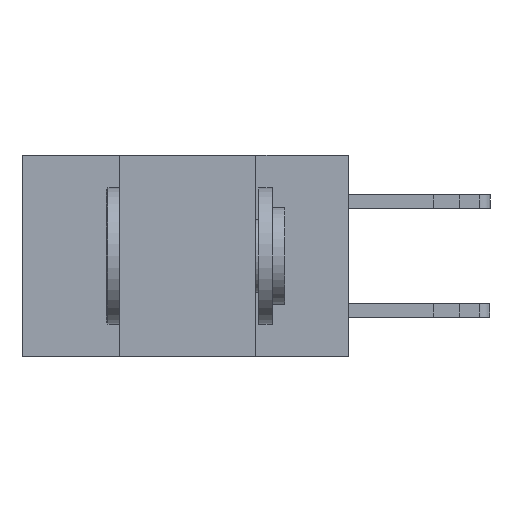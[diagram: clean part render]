
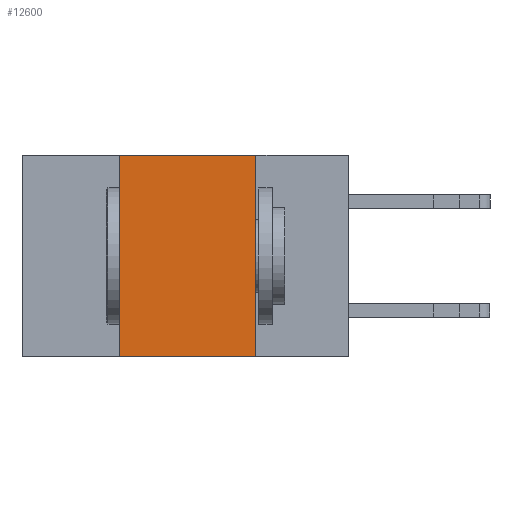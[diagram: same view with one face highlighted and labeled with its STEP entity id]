
A CAD part, left-side view. The second image highlights one B-rep face of the part: STEP entity #12600.
In plain terms, the highlighted planar face has unit normal (-1, 0, 0).
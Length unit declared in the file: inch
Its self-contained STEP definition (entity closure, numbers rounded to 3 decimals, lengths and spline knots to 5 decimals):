
#1509 = EDGE_CURVE ( 'NONE', #14684, #24895, #2768, .T. ) ;
#1620 = CARTESIAN_POINT ( 'NONE',  ( 0., 0.6, -0.37 ) ) ;
#1804 = AXIS2_PLACEMENT_3D ( 'NONE', #2085, #16652, #4203 ) ;
#2085 = CARTESIAN_POINT ( 'NONE',  ( 0., 0.6, 0. ) ) ;
#2451 = DIRECTION ( 'NONE',  ( 0., 0., -1. ) ) ;
#2768 = LINE ( 'NONE', #10231, #18687 ) ;
#2786 = VECTOR ( 'NONE', #5825, 39.37008 ) ;
#4203 = DIRECTION ( 'NONE',  ( 0., 0., -1. ) ) ;
#4285 = LINE ( 'NONE', #4635, #13384 ) ;
#4635 = CARTESIAN_POINT ( 'NONE',  ( 0., 0.6, 0. ) ) ;
#5825 = DIRECTION ( 'NONE',  ( 0., -1., 0. ) ) ;
#6370 = VECTOR ( 'NONE', #17420, 39.37008 ) ;
#7009 = CARTESIAN_POINT ( 'NONE',  ( 0., 0.42, 0. ) ) ;
#7042 = LINE ( 'NONE', #23529, #6370 ) ;
#7536 = EDGE_LOOP ( 'NONE', ( #23063, #16572, #15655, #19479 ) ) ;
#8328 = LINE ( 'NONE', #1620, #2786 ) ;
#10231 = CARTESIAN_POINT ( 'NONE',  ( 0., 0.17, 0. ) ) ;
#10263 = CARTESIAN_POINT ( 'NONE',  ( 0., 0.17, -0.37 ) ) ;
#12600 = ADVANCED_FACE ( 'NONE', ( #15675 ), #24826, .F. ) ;
#12912 = DIRECTION ( 'NONE',  ( 0., -1., 0. ) ) ;
#13384 = VECTOR ( 'NONE', #12912, 39.37008 ) ;
#14684 = VERTEX_POINT ( 'NONE', #23320 ) ;
#15655 = ORIENTED_EDGE ( 'NONE', *, *, #23907, .F. ) ;
#15675 = FACE_OUTER_BOUND ( 'NONE', #7536, .T. ) ;
#15969 = CARTESIAN_POINT ( 'NONE',  ( 0., 0.42, -0.37 ) ) ;
#16572 = ORIENTED_EDGE ( 'NONE', *, *, #20090, .F. ) ;
#16617 = VERTEX_POINT ( 'NONE', #15969 ) ;
#16652 = DIRECTION ( 'NONE',  ( 1., 0., 0. ) ) ;
#17420 = DIRECTION ( 'NONE',  ( 0., 0., 1. ) ) ;
#18687 = VECTOR ( 'NONE', #2451, 39.37008 ) ;
#19479 = ORIENTED_EDGE ( 'NONE', *, *, #19797, .T. ) ;
#19797 = EDGE_CURVE ( 'NONE', #16617, #24895, #8328, .T. ) ;
#20090 = EDGE_CURVE ( 'NONE', #25780, #14684, #4285, .T. ) ;
#23063 = ORIENTED_EDGE ( 'NONE', *, *, #1509, .F. ) ;
#23320 = CARTESIAN_POINT ( 'NONE',  ( 0., 0.17, 0. ) ) ;
#23529 = CARTESIAN_POINT ( 'NONE',  ( 0., 0.42, 0. ) ) ;
#23907 = EDGE_CURVE ( 'NONE', #16617, #25780, #7042, .T. ) ;
#24826 = PLANE ( 'NONE',  #1804 ) ;
#24895 = VERTEX_POINT ( 'NONE', #10263 ) ;
#25780 = VERTEX_POINT ( 'NONE', #7009 ) ;
